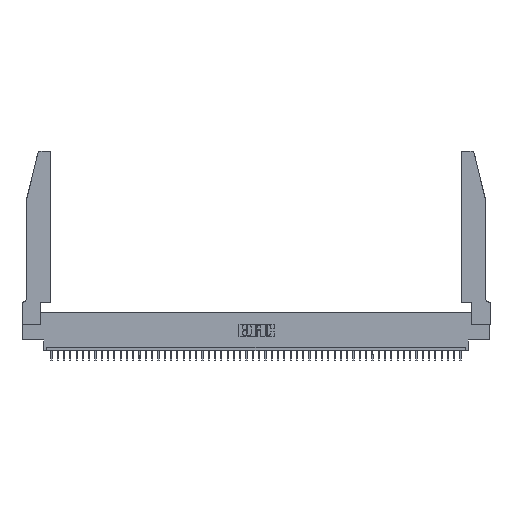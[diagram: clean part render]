
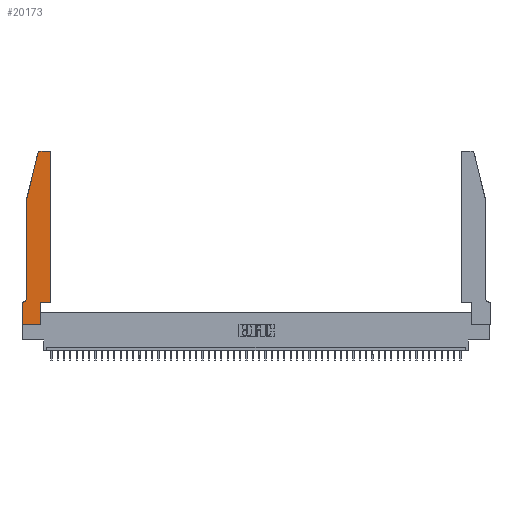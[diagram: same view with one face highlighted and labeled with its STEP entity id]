
A CAD part, top view. The second image highlights one B-rep face of the part: STEP entity #20173.
In plain terms, the highlighted planar face has unit normal (0, 0, 1).
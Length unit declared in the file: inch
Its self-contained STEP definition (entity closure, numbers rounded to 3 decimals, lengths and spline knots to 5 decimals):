
#310 = VERTEX_POINT ( 'NONE', #23910 ) ;
#2270 = VERTEX_POINT ( 'NONE', #15534 ) ;
#2530 = VERTEX_POINT ( 'NONE', #22455 ) ;
#2826 = EDGE_CURVE ( 'NONE', #2270, #8687, #22025, .T. ) ;
#3053 = DIRECTION ( 'NONE',  ( 0., 0., 1. ) ) ;
#3562 = VECTOR ( 'NONE', #28223, 39.37008 ) ;
#4543 = DIRECTION ( 'NONE',  ( 1., 0., 0. ) ) ;
#6333 = EDGE_CURVE ( 'NONE', #11638, #15814, #31625, .T. ) ;
#6929 = VECTOR ( 'NONE', #16039, 39.37008 ) ;
#6962 = CARTESIAN_POINT ( 'NONE',  ( 0.2865, 0.35, 0.37 ) ) ;
#7272 = LINE ( 'NONE', #40605, #3562 ) ;
#7832 = CARTESIAN_POINT ( 'NONE',  ( 0., 0., 0.37 ) ) ;
#8416 = FACE_OUTER_BOUND ( 'NONE', #9314, .T. ) ;
#8607 = VECTOR ( 'NONE', #21605, 39.37008 ) ;
#8687 = VERTEX_POINT ( 'NONE', #46775 ) ;
#8794 = CARTESIAN_POINT ( 'NONE',  ( 0., 0., 0.37 ) ) ;
#9193 = DIRECTION ( 'NONE',  ( 0., 0., -1. ) ) ;
#9314 = EDGE_LOOP ( 'NONE', ( #35859, #10536, #45279, #32904, #42799, #17233, #14692, #36628, #28333, #35186, #35185, #37129 ) ) ;
#10052 = CARTESIAN_POINT ( 'NONE',  ( 0.0755, 0.35, 0.37 ) ) ;
#10536 = ORIENTED_EDGE ( 'NONE', *, *, #30805, .T. ) ;
#10849 = AXIS2_PLACEMENT_3D ( 'NONE', #23088, #19286, #39696 ) ;
#11109 = CARTESIAN_POINT ( 'NONE',  ( 0.25487, 2.72718, 0.37 ) ) ;
#11638 = VERTEX_POINT ( 'NONE', #11109 ) ;
#11891 = EDGE_CURVE ( 'NONE', #15814, #14898, #17463, .T. ) ;
#11966 = CIRCLE ( 'NONE', #16724, 0.03 ) ;
#12037 = EDGE_CURVE ( 'NONE', #48599, #42861, #45423, .T. ) ;
#12335 = DIRECTION ( 'NONE',  ( 0., 1., 0. ) ) ;
#14235 = EDGE_CURVE ( 'NONE', #46481, #2270, #45714, .T. ) ;
#14634 = DIRECTION ( 'NONE',  ( -0.239, -0.971, 0. ) ) ;
#14692 = ORIENTED_EDGE ( 'NONE', *, *, #12037, .T. ) ;
#14898 = VERTEX_POINT ( 'NONE', #37056 ) ;
#15534 = CARTESIAN_POINT ( 'NONE',  ( 0.4205, 2.75, 0.37 ) ) ;
#15746 = CARTESIAN_POINT ( 'NONE',  ( 0.284, 2.72, 0.37 ) ) ;
#15814 = VERTEX_POINT ( 'NONE', #34104 ) ;
#16039 = DIRECTION ( 'NONE',  ( 0., -1., 0. ) ) ;
#16091 = VECTOR ( 'NONE', #14634, 39.37008 ) ;
#16724 = AXIS2_PLACEMENT_3D ( 'NONE', #15746, #19720, #23692 ) ;
#17233 = ORIENTED_EDGE ( 'NONE', *, *, #18753, .T. ) ;
#17463 = LINE ( 'NONE', #41899, #29875 ) ;
#18609 = CARTESIAN_POINT ( 'NONE',  ( 0., 0.35, 0.37 ) ) ;
#18753 = EDGE_CURVE ( 'NONE', #29679, #48599, #48983, .T. ) ;
#19286 = DIRECTION ( 'NONE',  ( 0., 0., 1. ) ) ;
#19456 = CARTESIAN_POINT ( 'NONE',  ( 0.2605, 2.75, 0.37 ) ) ;
#19720 = DIRECTION ( 'NONE',  ( 0., 0., 1. ) ) ;
#19749 = EDGE_CURVE ( 'NONE', #310, #2530, #7272, .T. ) ;
#20173 = ADVANCED_FACE ( 'NONE', ( #8416 ), #22218, .T. ) ;
#21605 = DIRECTION ( 'NONE',  ( -1., 0., 0. ) ) ;
#22025 = LINE ( 'NONE', #19456, #47017 ) ;
#22218 = PLANE ( 'NONE',  #23895 ) ;
#22432 = CIRCLE ( 'NONE', #42968, 0.07 ) ;
#22455 = CARTESIAN_POINT ( 'NONE',  ( 0.4505, 0.35, 0.37 ) ) ;
#22992 = CARTESIAN_POINT ( 'NONE',  ( 0., 0., 0.37 ) ) ;
#23088 = CARTESIAN_POINT ( 'NONE',  ( 0.4205, 2.72, 0.37 ) ) ;
#23416 = DIRECTION ( 'NONE',  ( 1., 0., 0. ) ) ;
#23692 = DIRECTION ( 'NONE',  ( 1., 0., 0. ) ) ;
#23895 = AXIS2_PLACEMENT_3D ( 'NONE', #18609, #3053, #4543 ) ;
#23896 = CARTESIAN_POINT ( 'NONE',  ( 0.0055, 0.35, 0.37 ) ) ;
#23910 = CARTESIAN_POINT ( 'NONE',  ( 0.2865, 0.35, 0.37 ) ) ;
#26070 = EDGE_CURVE ( 'NONE', #43419, #310, #31710, .T. ) ;
#26564 = CARTESIAN_POINT ( 'NONE',  ( 0.0755, 2., 0.37 ) ) ;
#27404 = VECTOR ( 'NONE', #50431, 39.37008 ) ;
#28223 = DIRECTION ( 'NONE',  ( 1., 0., 0. ) ) ;
#28333 = ORIENTED_EDGE ( 'NONE', *, *, #26070, .T. ) ;
#28714 = VECTOR ( 'NONE', #23416, 39.37008 ) ;
#29679 = VERTEX_POINT ( 'NONE', #23896 ) ;
#29875 = VECTOR ( 'NONE', #41707, 39.37008 ) ;
#29973 = LINE ( 'NONE', #38846, #42462 ) ;
#30741 = EDGE_CURVE ( 'NONE', #2530, #46481, #29973, .T. ) ;
#30805 = EDGE_CURVE ( 'NONE', #8687, #11638, #11966, .T. ) ;
#31625 = LINE ( 'NONE', #26564, #16091 ) ;
#31710 = LINE ( 'NONE', #6962, #27404 ) ;
#32904 = ORIENTED_EDGE ( 'NONE', *, *, #11891, .T. ) ;
#32965 = CARTESIAN_POINT ( 'NONE',  ( 0.0055, 0.42, 0.37 ) ) ;
#34104 = CARTESIAN_POINT ( 'NONE',  ( 0.0755, 2., 0.37 ) ) ;
#35185 = ORIENTED_EDGE ( 'NONE', *, *, #30741, .T. ) ;
#35186 = ORIENTED_EDGE ( 'NONE', *, *, #19749, .T. ) ;
#35275 = DIRECTION ( 'NONE',  ( -1., 0., 0. ) ) ;
#35859 = ORIENTED_EDGE ( 'NONE', *, *, #2826, .T. ) ;
#36628 = ORIENTED_EDGE ( 'NONE', *, *, #40934, .T. ) ;
#36972 = DIRECTION ( 'NONE',  ( -1., 0., 0. ) ) ;
#37056 = CARTESIAN_POINT ( 'NONE',  ( 0.0755, 0.42, 0.37 ) ) ;
#37129 = ORIENTED_EDGE ( 'NONE', *, *, #14235, .T. ) ;
#38087 = LINE ( 'NONE', #7832, #28714 ) ;
#38846 = CARTESIAN_POINT ( 'NONE',  ( 0.4505, 0.35, 0.37 ) ) ;
#39696 = DIRECTION ( 'NONE',  ( 1., 0., 0. ) ) ;
#40605 = CARTESIAN_POINT ( 'NONE',  ( 0.4505, 0.35, 0.37 ) ) ;
#40892 = CARTESIAN_POINT ( 'NONE',  ( 0.2865, 0., 0.37 ) ) ;
#40934 = EDGE_CURVE ( 'NONE', #42861, #43419, #38087, .T. ) ;
#41707 = DIRECTION ( 'NONE',  ( 0., -1., 0. ) ) ;
#41899 = CARTESIAN_POINT ( 'NONE',  ( 0.0755, 2., 0.37 ) ) ;
#42462 = VECTOR ( 'NONE', #12335, 39.37008 ) ;
#42771 = CARTESIAN_POINT ( 'NONE',  ( 0., 0.35, 0.37 ) ) ;
#42799 = ORIENTED_EDGE ( 'NONE', *, *, #50285, .T. ) ;
#42861 = VERTEX_POINT ( 'NONE', #8794 ) ;
#42968 = AXIS2_PLACEMENT_3D ( 'NONE', #32965, #9193, #36972 ) ;
#43419 = VERTEX_POINT ( 'NONE', #40892 ) ;
#45279 = ORIENTED_EDGE ( 'NONE', *, *, #6333, .T. ) ;
#45423 = LINE ( 'NONE', #22992, #6929 ) ;
#45714 = CIRCLE ( 'NONE', #10849, 0.03 ) ;
#46481 = VERTEX_POINT ( 'NONE', #50689 ) ;
#46775 = CARTESIAN_POINT ( 'NONE',  ( 0.284, 2.75, 0.37 ) ) ;
#47017 = VECTOR ( 'NONE', #35275, 39.37008 ) ;
#48599 = VERTEX_POINT ( 'NONE', #42771 ) ;
#48983 = LINE ( 'NONE', #10052, #8607 ) ;
#50285 = EDGE_CURVE ( 'NONE', #14898, #29679, #22432, .T. ) ;
#50431 = DIRECTION ( 'NONE',  ( 0., 1., 0. ) ) ;
#50689 = CARTESIAN_POINT ( 'NONE',  ( 0.4505, 2.72, 0.37 ) ) ;
